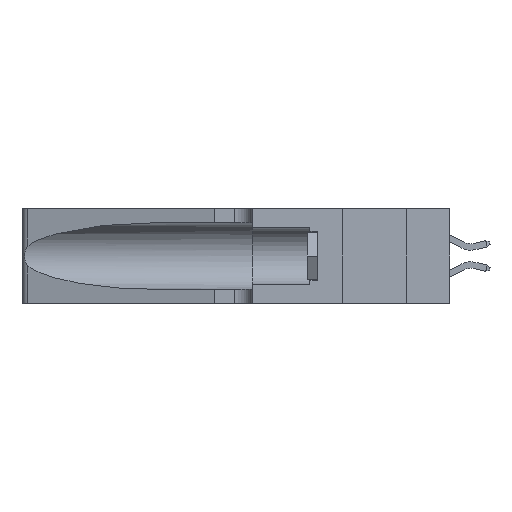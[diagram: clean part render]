
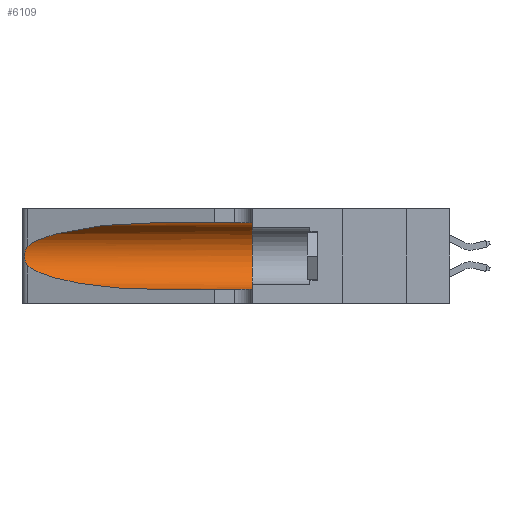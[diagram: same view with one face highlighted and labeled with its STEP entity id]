
A CAD part, left-side view. The second image highlights one B-rep face of the part: STEP entity #6109.
In plain terms, the highlighted cylindrical face has radius 3.308 mm (diameter 6.617 mm), a partial arc.
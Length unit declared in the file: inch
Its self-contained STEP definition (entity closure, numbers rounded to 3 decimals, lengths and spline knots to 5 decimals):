
#560 = AXIS2_PLACEMENT_3D ( 'NONE', #22769, #11122, #27483 ) ;
#630 = CARTESIAN_POINT ( 'NONE',  ( 0.25555, 1.22994, 0.2215 ) ) ;
#1139 = CARTESIAN_POINT ( 'NONE',  ( 0.25487, 1.22718, 0.22369 ) ) ;
#1530 = DIRECTION ( 'NONE',  ( 0., 0., 1. ) ) ;
#2957 = CARTESIAN_POINT ( 'NONE',  ( 0.1305, 1.61858, 0.31525 ) ) ;
#2971 = CARTESIAN_POINT ( 'NONE',  ( 0.25787, 1.23484, 0.2124 ) ) ;
#3106 = VERTEX_POINT ( 'NONE', #19443 ) ;
#4986 = LINE ( 'NONE', #2957, #29157 ) ;
#5207 = EDGE_CURVE ( 'NONE', #15612, #17907, #25151, .T. ) ;
#5325 = CARTESIAN_POINT ( 'NONE',  ( 0.26018, 1.23835, 0.19895 ) ) ;
#6109 = ADVANCED_FACE ( 'NONE', ( #27375 ), #26646, .F. ) ;
#7005 = ORIENTED_EDGE ( 'NONE', *, *, #5207, .T. ) ;
#7028 = CARTESIAN_POINT ( 'NONE',  ( 0.25487, 1.22718, 0.14631 ) ) ;
#7200 = CIRCLE ( 'NONE', #15958, 0.13025 ) ;
#7451 = CARTESIAN_POINT ( 'NONE',  ( 0.1305, 0.72297, 0.31525 ) ) ;
#7687 = CARTESIAN_POINT ( 'NONE',  ( 0.26075, 1.23896, 0.178 ) ) ;
#8662 = VERTEX_POINT ( 'NONE', #20165 ) ;
#9725 = VERTEX_POINT ( 'NONE', #20438 ) ;
#10034 = CARTESIAN_POINT ( 'NONE',  ( 0.25856, 1.23593, 0.16098 ) ) ;
#10255 = CARTESIAN_POINT ( 'NONE',  ( 0.1305, 1.61858, 0.05475 ) ) ;
#11122 = DIRECTION ( 'NONE',  ( 0., -1., 0. ) ) ;
#11180 = EDGE_CURVE ( 'NONE', #17907, #8662, #19157, .T. ) ;
#11804 = CARTESIAN_POINT ( 'NONE',  ( 0.25487, 1.22718, 0.22369 ) ) ;
#11871 = CARTESIAN_POINT ( 'NONE',  ( 0.1305, 0.72297, 0.05475 ) ) ;
#12388 = CARTESIAN_POINT ( 'NONE',  ( 0.25639, 1.23186, 0.15144 ) ) ;
#12500 = EDGE_CURVE ( 'NONE', #19289, #15612, #18770, .T. ) ;
#14628 = EDGE_LOOP ( 'NONE', ( #21003, #7005, #20545, #21616, #18971, #20047 ) ) ;
#14736 = CARTESIAN_POINT ( 'NONE',  ( 0.25487, 1.22718, 0.14631 ) ) ;
#15516 = DIRECTION ( 'NONE',  ( 0., 1., 0. ) ) ;
#15612 = VERTEX_POINT ( 'NONE', #1139 ) ;
#15958 = AXIS2_PLACEMENT_3D ( 'NONE', #29534, #15516, #1530 ) ;
#16482 = CARTESIAN_POINT ( 'NONE',  ( 0.2373, 1.15595, 0.08982 ) ) ;
#16972 = CARTESIAN_POINT ( 'NONE',  ( 0.25639, 1.23184, 0.21858 ) ) ;
#17757 = EDGE_CURVE ( 'NONE', #9725, #3106, #7200, .T. ) ;
#17907 = VERTEX_POINT ( 'NONE', #7028 ) ;
#18770 =( BOUNDED_CURVE ( )  B_SPLINE_CURVE ( 3, ( #21096, #23461, #25808, #11804 ),
 .UNSPECIFIED., .F., .F. ) 
 B_SPLINE_CURVE_WITH_KNOTS ( ( 4, 4 ),
 ( 1.5708, 2.84003 ),
 .UNSPECIFIED. ) 
 CURVE ( )  GEOMETRIC_REPRESENTATION_ITEM ( )  RATIONAL_B_SPLINE_CURVE ( ( 1., 0.87, 0.87, 1. ) ) 
 REPRESENTATION_ITEM ( '' )  );
#18813 = CARTESIAN_POINT ( 'NONE',  ( 0.25487, 1.22718, 0.14631 ) ) ;
#18971 = ORIENTED_EDGE ( 'NONE', *, *, #17757, .F. ) ;
#19116 = LINE ( 'NONE', #10255, #24617 ) ;
#19157 =( BOUNDED_CURVE ( )  B_SPLINE_CURVE ( 3, ( #18813, #16482, #25880, #11871 ),
 .UNSPECIFIED., .F., .F. ) 
 B_SPLINE_CURVE_WITH_KNOTS ( ( 4, 4 ),
 ( 3.44316, 4.71239 ),
 .UNSPECIFIED. ) 
 CURVE ( )  GEOMETRIC_REPRESENTATION_ITEM ( )  RATIONAL_B_SPLINE_CURVE ( ( 1., 0.87, 0.87, 1. ) ) 
 REPRESENTATION_ITEM ( '' )  );
#19289 = VERTEX_POINT ( 'NONE', #7451 ) ;
#19341 = CARTESIAN_POINT ( 'NONE',  ( 0.25854, 1.2359, 0.20912 ) ) ;
#19443 = CARTESIAN_POINT ( 'NONE',  ( 0.1305, 0.35, 0.05475 ) ) ;
#20047 = ORIENTED_EDGE ( 'NONE', *, *, #27512, .F. ) ;
#20165 = CARTESIAN_POINT ( 'NONE',  ( 0.1305, 0.72297, 0.05475 ) ) ;
#20438 = CARTESIAN_POINT ( 'NONE',  ( 0.1305, 0.35, 0.31525 ) ) ;
#20545 = ORIENTED_EDGE ( 'NONE', *, *, #11180, .T. ) ;
#21003 = ORIENTED_EDGE ( 'NONE', *, *, #12500, .T. ) ;
#21096 = CARTESIAN_POINT ( 'NONE',  ( 0.1305, 0.72297, 0.31525 ) ) ;
#21590 = CARTESIAN_POINT ( 'NONE',  ( 0.25487, 1.22718, 0.22369 ) ) ;
#21616 = ORIENTED_EDGE ( 'NONE', *, *, #22212, .T. ) ;
#21684 = CARTESIAN_POINT ( 'NONE',  ( 0.26075, 1.23896, 0.19203 ) ) ;
#22212 = EDGE_CURVE ( 'NONE', #8662, #3106, #19116, .T. ) ;
#22769 = CARTESIAN_POINT ( 'NONE',  ( 0.1305, 1.61858, 0.185 ) ) ;
#23461 = CARTESIAN_POINT ( 'NONE',  ( 0.18966, 0.96281, 0.31525 ) ) ;
#24033 = CARTESIAN_POINT ( 'NONE',  ( 0.26017, 1.23833, 0.17102 ) ) ;
#24255 = DIRECTION ( 'NONE',  ( 0., -1., 0. ) ) ;
#24617 = VECTOR ( 'NONE', #24255, 39.37008 ) ;
#25151 = B_SPLINE_CURVE_WITH_KNOTS ( 'NONE', 3,
 ( #21590, #630, #16972, #2971, #19341, #5325, #21684, #7687, #24033, #10034, #26400, #12388, #28745, #14736 ),
 .UNSPECIFIED., .F., .F.,
 ( 4, 2, 2, 2, 2, 2, 4 ),
 ( 0., 0.00027, 0.00053, 0.00107, 0.0016, 0.00187, 0.00214 ),
 .UNSPECIFIED. ) ;
#25808 = CARTESIAN_POINT ( 'NONE',  ( 0.2373, 1.15595, 0.28018 ) ) ;
#25880 = CARTESIAN_POINT ( 'NONE',  ( 0.18966, 0.96281, 0.05475 ) ) ;
#26400 = CARTESIAN_POINT ( 'NONE',  ( 0.25789, 1.23486, 0.15765 ) ) ;
#26646 = CYLINDRICAL_SURFACE ( 'NONE', #560, 0.13025 ) ;
#27375 = FACE_OUTER_BOUND ( 'NONE', #14628, .T. ) ;
#27483 = DIRECTION ( 'NONE',  ( 0., 0., -1. ) ) ;
#27512 = EDGE_CURVE ( 'NONE', #19289, #9725, #4986, .T. ) ;
#28725 = DIRECTION ( 'NONE',  ( 0., -1., 0. ) ) ;
#28745 = CARTESIAN_POINT ( 'NONE',  ( 0.25555, 1.22993, 0.14849 ) ) ;
#29157 = VECTOR ( 'NONE', #28725, 39.37008 ) ;
#29534 = CARTESIAN_POINT ( 'NONE',  ( 0.1305, 0.35, 0.185 ) ) ;
